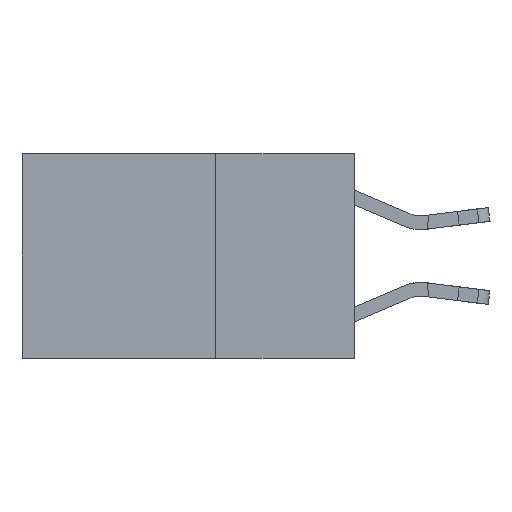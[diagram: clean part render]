
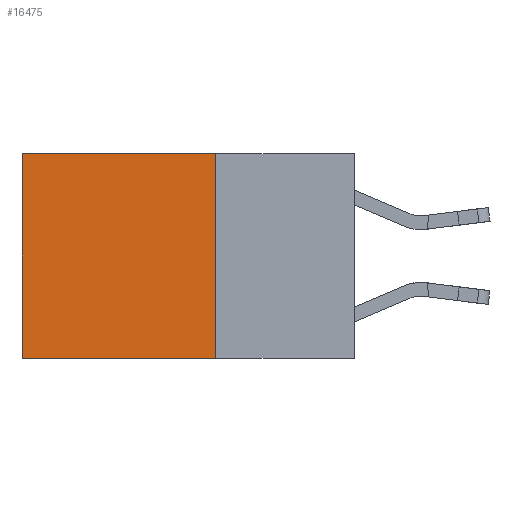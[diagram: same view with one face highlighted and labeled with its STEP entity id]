
A CAD part, left-side view. The second image highlights one B-rep face of the part: STEP entity #16475.
In plain terms, the highlighted planar face has unit normal (-1, 0, 0).
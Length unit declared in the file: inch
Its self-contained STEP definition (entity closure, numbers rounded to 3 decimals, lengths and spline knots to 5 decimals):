
#486 = CARTESIAN_POINT ( 'NONE',  ( 0.2625, 0.25, 0. ) ) ;
#681 = CARTESIAN_POINT ( 'NONE',  ( 0.2625, 0.25, -0.37 ) ) ;
#1479 = LINE ( 'NONE', #14155, #8408 ) ;
#2640 = DIRECTION ( 'NONE',  ( 0., 0., -1. ) ) ;
#3494 = VERTEX_POINT ( 'NONE', #9362 ) ;
#4183 = CARTESIAN_POINT ( 'NONE',  ( 0.2625, 0.6, 0. ) ) ;
#4191 = CARTESIAN_POINT ( 'NONE',  ( 0.2625, 0.25, -0.37 ) ) ;
#4310 = LINE ( 'NONE', #13109, #5871 ) ;
#5646 = DIRECTION ( 'NONE',  ( 0., 1., 0. ) ) ;
#5871 = VECTOR ( 'NONE', #21887, 39.37008 ) ;
#6936 = EDGE_LOOP ( 'NONE', ( #24570, #12659, #17516, #20297 ) ) ;
#7432 = AXIS2_PLACEMENT_3D ( 'NONE', #486, #18210, #2640 ) ;
#8408 = VECTOR ( 'NONE', #5646, 39.37008 ) ;
#8536 = DIRECTION ( 'NONE',  ( 0., 1., 0. ) ) ;
#8930 = EDGE_CURVE ( 'NONE', #26399, #26920, #23326, .T. ) ;
#9362 = CARTESIAN_POINT ( 'NONE',  ( 0.2625, 0.6, -0.37 ) ) ;
#10620 = EDGE_CURVE ( 'NONE', #18863, #3494, #4310, .T. ) ;
#12659 = ORIENTED_EDGE ( 'NONE', *, *, #25539, .F. ) ;
#13109 = CARTESIAN_POINT ( 'NONE',  ( 0.2625, 0.6, 0. ) ) ;
#14155 = CARTESIAN_POINT ( 'NONE',  ( 0.2625, 0.25, 0. ) ) ;
#14843 = DIRECTION ( 'NONE',  ( 0., 0., -1. ) ) ;
#16475 = ADVANCED_FACE ( 'NONE', ( #20083 ), #22522, .F. ) ;
#17516 = ORIENTED_EDGE ( 'NONE', *, *, #8930, .F. ) ;
#18210 = DIRECTION ( 'NONE',  ( 1., 0., 0. ) ) ;
#18722 = CARTESIAN_POINT ( 'NONE',  ( 0.2625, 0.25, 0. ) ) ;
#18863 = VERTEX_POINT ( 'NONE', #4183 ) ;
#19483 = LINE ( 'NONE', #4191, #24261 ) ;
#20022 = EDGE_CURVE ( 'NONE', #26399, #18863, #1479, .T. ) ;
#20083 = FACE_OUTER_BOUND ( 'NONE', #6936, .T. ) ;
#20297 = ORIENTED_EDGE ( 'NONE', *, *, #20022, .T. ) ;
#21052 = VECTOR ( 'NONE', #14843, 39.37008 ) ;
#21887 = DIRECTION ( 'NONE',  ( 0., 0., -1. ) ) ;
#22522 = PLANE ( 'NONE',  #7432 ) ;
#23326 = LINE ( 'NONE', #23617, #21052 ) ;
#23617 = CARTESIAN_POINT ( 'NONE',  ( 0.2625, 0.25, 0. ) ) ;
#24261 = VECTOR ( 'NONE', #8536, 39.37008 ) ;
#24570 = ORIENTED_EDGE ( 'NONE', *, *, #10620, .T. ) ;
#25539 = EDGE_CURVE ( 'NONE', #26920, #3494, #19483, .T. ) ;
#26399 = VERTEX_POINT ( 'NONE', #18722 ) ;
#26920 = VERTEX_POINT ( 'NONE', #681 ) ;
